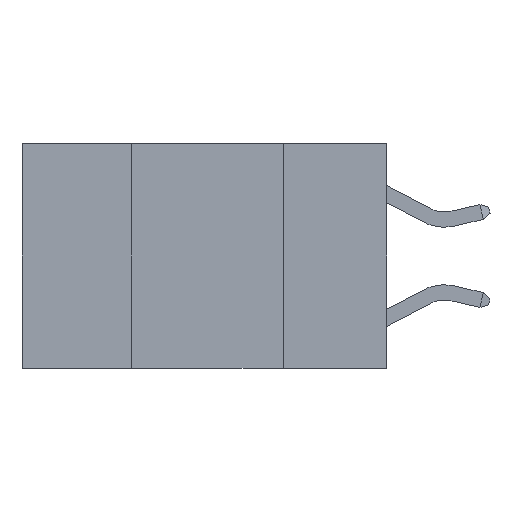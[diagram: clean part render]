
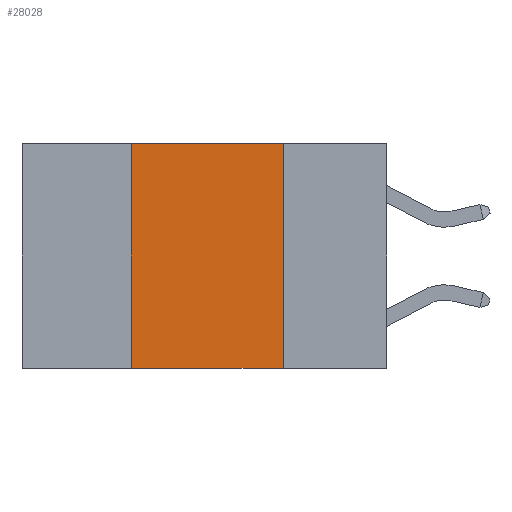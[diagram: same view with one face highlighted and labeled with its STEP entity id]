
A CAD part, left-side view. The second image highlights one B-rep face of the part: STEP entity #28028.
In plain terms, the highlighted planar face has unit normal (-1, 0, 0).
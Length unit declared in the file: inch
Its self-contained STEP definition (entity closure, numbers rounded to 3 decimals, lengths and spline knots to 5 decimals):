
#1488 = DIRECTION ( 'NONE',  ( 0., -1., 0. ) ) ;
#2033 = DIRECTION ( 'NONE',  ( 0., -1., 0. ) ) ;
#2140 = CARTESIAN_POINT ( 'NONE',  ( 0., 0.6, 0. ) ) ;
#3956 = EDGE_CURVE ( 'NONE', #14723, #15696, #20588, .T. ) ;
#5397 = LINE ( 'NONE', #7460, #10868 ) ;
#6144 = DIRECTION ( 'NONE',  ( 0., 0., -1. ) ) ;
#6511 = CARTESIAN_POINT ( 'NONE',  ( 0., 0.17, 0. ) ) ;
#6878 = VECTOR ( 'NONE', #1488, 39.37008 ) ;
#7460 = CARTESIAN_POINT ( 'NONE',  ( 0., 0.42, 0. ) ) ;
#7915 = CARTESIAN_POINT ( 'NONE',  ( 0., 0.42, 0. ) ) ;
#8653 = VERTEX_POINT ( 'NONE', #13777 ) ;
#9592 = ORIENTED_EDGE ( 'NONE', *, *, #10447, .F. ) ;
#10447 = EDGE_CURVE ( 'NONE', #15696, #8653, #15848, .T. ) ;
#10481 = DIRECTION ( 'NONE',  ( 1., 0., 0. ) ) ;
#10868 = VECTOR ( 'NONE', #28500, 39.37008 ) ;
#12491 = ORIENTED_EDGE ( 'NONE', *, *, #12985, .T. ) ;
#12985 = EDGE_CURVE ( 'NONE', #27276, #8653, #18598, .T. ) ;
#13592 = VECTOR ( 'NONE', #2033, 39.37008 ) ;
#13777 = CARTESIAN_POINT ( 'NONE',  ( 0., 0.17, -0.37 ) ) ;
#14723 = VERTEX_POINT ( 'NONE', #7915 ) ;
#14841 = CARTESIAN_POINT ( 'NONE',  ( 0., 0.42, -0.37 ) ) ;
#15311 = EDGE_LOOP ( 'NONE', ( #9592, #28962, #17302, #12491 ) ) ;
#15696 = VERTEX_POINT ( 'NONE', #6511 ) ;
#15848 = LINE ( 'NONE', #17812, #27524 ) ;
#17302 = ORIENTED_EDGE ( 'NONE', *, *, #22423, .F. ) ;
#17623 = AXIS2_PLACEMENT_3D ( 'NONE', #22052, #10481, #26849 ) ;
#17812 = CARTESIAN_POINT ( 'NONE',  ( 0., 0.17, 0. ) ) ;
#18598 = LINE ( 'NONE', #22678, #6878 ) ;
#20588 = LINE ( 'NONE', #2140, #13592 ) ;
#22052 = CARTESIAN_POINT ( 'NONE',  ( 0., 0.6, 0. ) ) ;
#22423 = EDGE_CURVE ( 'NONE', #27276, #14723, #5397, .T. ) ;
#22678 = CARTESIAN_POINT ( 'NONE',  ( 0., 0.6, -0.37 ) ) ;
#24504 = PLANE ( 'NONE',  #17623 ) ;
#26639 = FACE_OUTER_BOUND ( 'NONE', #15311, .T. ) ;
#26849 = DIRECTION ( 'NONE',  ( 0., 0., -1. ) ) ;
#27276 = VERTEX_POINT ( 'NONE', #14841 ) ;
#27524 = VECTOR ( 'NONE', #6144, 39.37008 ) ;
#28028 = ADVANCED_FACE ( 'NONE', ( #26639 ), #24504, .F. ) ;
#28500 = DIRECTION ( 'NONE',  ( 0., 0., 1. ) ) ;
#28962 = ORIENTED_EDGE ( 'NONE', *, *, #3956, .F. ) ;
